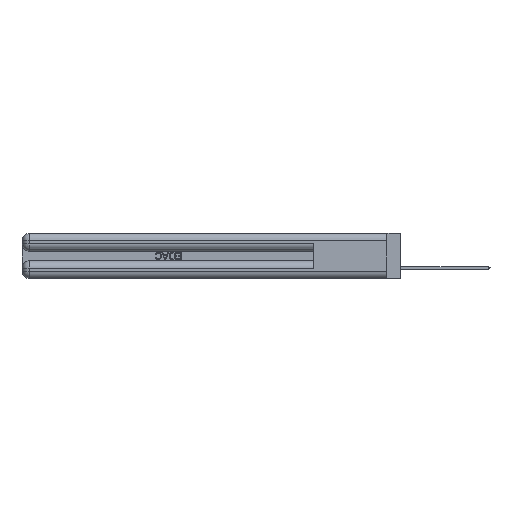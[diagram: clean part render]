
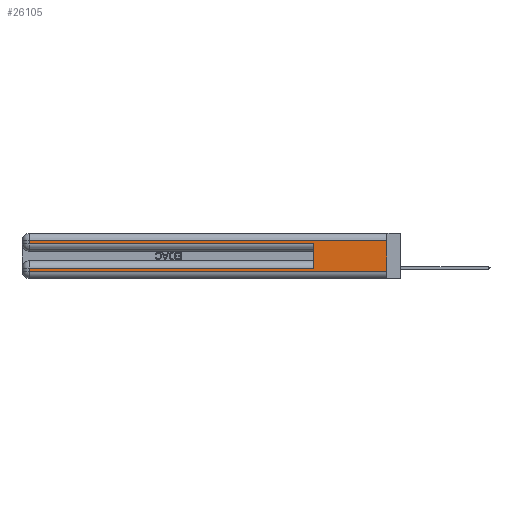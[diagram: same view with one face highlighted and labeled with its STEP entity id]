
A CAD part, left-side view. The second image highlights one B-rep face of the part: STEP entity #26105.
In plain terms, the highlighted planar face has unit normal (-1, 0, 0).
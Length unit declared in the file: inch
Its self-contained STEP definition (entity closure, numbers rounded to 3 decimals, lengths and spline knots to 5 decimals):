
#1948 = EDGE_CURVE ( 'NONE', #36853, #22752, #18665, .T. ) ;
#2511 = DIRECTION ( 'NONE',  ( 0., -1., 0. ) ) ;
#3918 = VECTOR ( 'NONE', #50810, 39.37008 ) ;
#4534 = FACE_OUTER_BOUND ( 'NONE', #49826, .T. ) ;
#5124 = CARTESIAN_POINT ( 'NONE',  ( 0., 0., 0.085 ) ) ;
#5389 = DIRECTION ( 'NONE',  ( 0., 0., -1. ) ) ;
#5885 = VERTEX_POINT ( 'NONE', #46291 ) ;
#6097 = LINE ( 'NONE', #40196, #14486 ) ;
#6505 = CARTESIAN_POINT ( 'NONE',  ( 0., 0.6, 0.085 ) ) ;
#8449 = CARTESIAN_POINT ( 'NONE',  ( 0., 0., 0.37 ) ) ;
#9088 = VERTEX_POINT ( 'NONE', #51558 ) ;
#9610 = DIRECTION ( 'NONE',  ( 0., 0., -1. ) ) ;
#9645 = CARTESIAN_POINT ( 'NONE',  ( 0., 0., 0.06 ) ) ;
#9700 = ORIENTED_EDGE ( 'NONE', *, *, #1948, .F. ) ;
#11261 = CARTESIAN_POINT ( 'NONE',  ( 0., 0., 0.31 ) ) ;
#14486 = VECTOR ( 'NONE', #15558, 39.37008 ) ;
#15558 = DIRECTION ( 'NONE',  ( 0., 0., -1. ) ) ;
#15730 = LINE ( 'NONE', #51338, #49954 ) ;
#16775 = ORIENTED_EDGE ( 'NONE', *, *, #22860, .T. ) ;
#17020 = DIRECTION ( 'NONE',  ( 0., 1., 0. ) ) ;
#17532 = CARTESIAN_POINT ( 'NONE',  ( 0., 0., 0.285 ) ) ;
#17933 = VERTEX_POINT ( 'NONE', #50510 ) ;
#18665 = LINE ( 'NONE', #8449, #3918 ) ;
#19199 = VECTOR ( 'NONE', #17020, 39.37008 ) ;
#19642 = VERTEX_POINT ( 'NONE', #44561 ) ;
#19756 = VECTOR ( 'NONE', #25459, 39.37008 ) ;
#20823 = ORIENTED_EDGE ( 'NONE', *, *, #42888, .T. ) ;
#21704 = ORIENTED_EDGE ( 'NONE', *, *, #33559, .T. ) ;
#22752 = VERTEX_POINT ( 'NONE', #9645 ) ;
#22860 = EDGE_CURVE ( 'NONE', #35339, #5885, #52089, .T. ) ;
#25082 = VECTOR ( 'NONE', #5389, 39.37008 ) ;
#25459 = DIRECTION ( 'NONE',  ( 0., 1., 0. ) ) ;
#25486 = DIRECTION ( 'NONE',  ( 1., 0., 0. ) ) ;
#25691 = LINE ( 'NONE', #42985, #25082 ) ;
#26105 = ADVANCED_FACE ( 'NONE', ( #4534 ), #33612, .F. ) ;
#26223 = VECTOR ( 'NONE', #46370, 39.37008 ) ;
#26427 = ORIENTED_EDGE ( 'NONE', *, *, #37115, .T. ) ;
#30203 = LINE ( 'NONE', #36997, #19199 ) ;
#31482 = CARTESIAN_POINT ( 'NONE',  ( 0., 0., 0.06 ) ) ;
#33457 = EDGE_CURVE ( 'NONE', #41105, #5885, #15730, .T. ) ;
#33559 = EDGE_CURVE ( 'NONE', #17933, #22752, #52523, .T. ) ;
#33612 = PLANE ( 'NONE',  #36162 ) ;
#33958 = CARTESIAN_POINT ( 'NONE',  ( 0., 0., 0.37 ) ) ;
#35339 = VERTEX_POINT ( 'NONE', #36470 ) ;
#35653 = ORIENTED_EDGE ( 'NONE', *, *, #47499, .T. ) ;
#36162 = AXIS2_PLACEMENT_3D ( 'NONE', #33958, #25486, #9610 ) ;
#36470 = CARTESIAN_POINT ( 'NONE',  ( 0., 2.94, 0.285 ) ) ;
#36853 = VERTEX_POINT ( 'NONE', #11261 ) ;
#36997 = CARTESIAN_POINT ( 'NONE',  ( 0., 0., 0.31 ) ) ;
#37115 = EDGE_CURVE ( 'NONE', #36853, #19642, #30203, .T. ) ;
#39458 = ORIENTED_EDGE ( 'NONE', *, *, #33457, .F. ) ;
#40196 = CARTESIAN_POINT ( 'NONE',  ( 0., 2.94, 0.37 ) ) ;
#41105 = VERTEX_POINT ( 'NONE', #6505 ) ;
#41490 = VECTOR ( 'NONE', #2511, 39.37008 ) ;
#42628 = DIRECTION ( 'NONE',  ( 0., 0., 1. ) ) ;
#42888 = EDGE_CURVE ( 'NONE', #19642, #35339, #6097, .T. ) ;
#42985 = CARTESIAN_POINT ( 'NONE',  ( 0., 2.94, 0.37 ) ) ;
#44561 = CARTESIAN_POINT ( 'NONE',  ( 0., 2.94, 0.31 ) ) ;
#45499 = EDGE_CURVE ( 'NONE', #9088, #17933, #25691, .T. ) ;
#46214 = LINE ( 'NONE', #5124, #19756 ) ;
#46291 = CARTESIAN_POINT ( 'NONE',  ( 0., 0.6, 0.285 ) ) ;
#46370 = DIRECTION ( 'NONE',  ( 0., -1., 0. ) ) ;
#47499 = EDGE_CURVE ( 'NONE', #41105, #9088, #46214, .T. ) ;
#48918 = ORIENTED_EDGE ( 'NONE', *, *, #45499, .T. ) ;
#49826 = EDGE_LOOP ( 'NONE', ( #9700, #26427, #20823, #16775, #39458, #35653, #48918, #21704 ) ) ;
#49954 = VECTOR ( 'NONE', #42628, 39.37008 ) ;
#50510 = CARTESIAN_POINT ( 'NONE',  ( 0., 2.94, 0.06 ) ) ;
#50810 = DIRECTION ( 'NONE',  ( 0., 0., -1. ) ) ;
#51338 = CARTESIAN_POINT ( 'NONE',  ( 0., 0.6, 0.145 ) ) ;
#51558 = CARTESIAN_POINT ( 'NONE',  ( 0., 2.94, 0.085 ) ) ;
#52089 = LINE ( 'NONE', #17532, #26223 ) ;
#52523 = LINE ( 'NONE', #31482, #41490 ) ;
